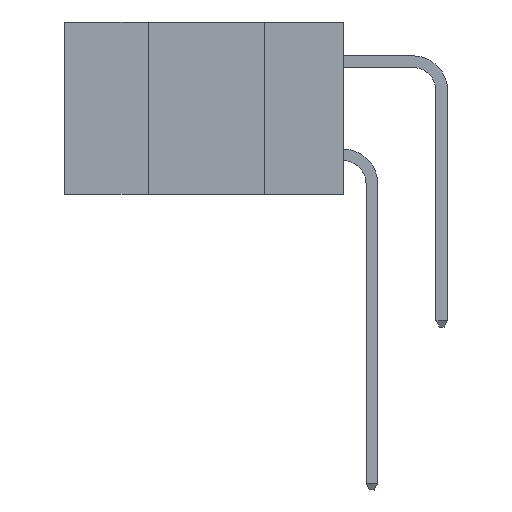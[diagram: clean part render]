
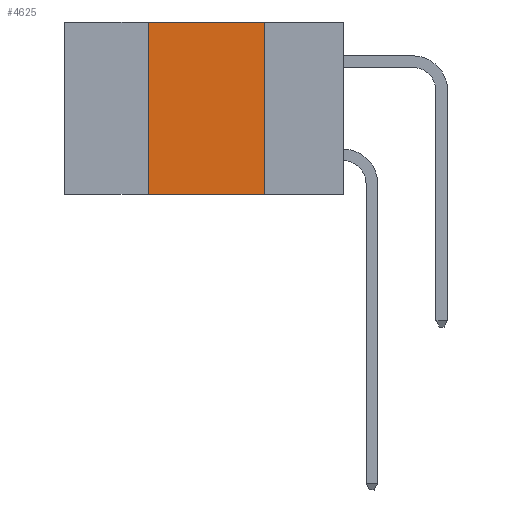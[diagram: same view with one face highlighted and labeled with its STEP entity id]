
A CAD part, left-side view. The second image highlights one B-rep face of the part: STEP entity #4625.
In plain terms, the highlighted planar face has unit normal (-1, 0, 0).
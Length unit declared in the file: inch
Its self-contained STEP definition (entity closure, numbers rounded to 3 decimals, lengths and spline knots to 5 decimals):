
#316 = LINE ( 'NONE', #6072, #7468 ) ;
#452 = EDGE_LOOP ( 'NONE', ( #10385, #9498, #10636, #984 ) ) ;
#498 = EDGE_CURVE ( 'NONE', #5081, #2629, #4426, .T. ) ;
#587 = CARTESIAN_POINT ( 'NONE',  ( 0., 0.42, 0. ) ) ;
#903 = DIRECTION ( 'NONE',  ( 1., 0., 0. ) ) ;
#962 = FACE_OUTER_BOUND ( 'NONE', #452, .T. ) ;
#984 = ORIENTED_EDGE ( 'NONE', *, *, #5746, .T. ) ;
#990 = CARTESIAN_POINT ( 'NONE',  ( 0., 0.6, 0. ) ) ;
#1086 = DIRECTION ( 'NONE',  ( 0., 0., -1. ) ) ;
#1478 = VECTOR ( 'NONE', #10584, 39.37008 ) ;
#1640 = PLANE ( 'NONE',  #8511 ) ;
#2348 = CARTESIAN_POINT ( 'NONE',  ( 0., 0.42, -0.37 ) ) ;
#2629 = VERTEX_POINT ( 'NONE', #8640 ) ;
#3432 = CARTESIAN_POINT ( 'NONE',  ( 0., 0.17, -0.37 ) ) ;
#3482 = CARTESIAN_POINT ( 'NONE',  ( 0., 0.6, -0.37 ) ) ;
#3766 = LINE ( 'NONE', #3482, #6515 ) ;
#3848 = CARTESIAN_POINT ( 'NONE',  ( 0., 0.42, 0. ) ) ;
#4426 = LINE ( 'NONE', #10821, #1478 ) ;
#4625 = ADVANCED_FACE ( 'NONE', ( #962 ), #1640, .F. ) ;
#5081 = VERTEX_POINT ( 'NONE', #587 ) ;
#5691 = VERTEX_POINT ( 'NONE', #2348 ) ;
#5729 = LINE ( 'NONE', #3848, #10146 ) ;
#5746 = EDGE_CURVE ( 'NONE', #5691, #7994, #3766, .T. ) ;
#6072 = CARTESIAN_POINT ( 'NONE',  ( 0., 0.17, 0. ) ) ;
#6515 = VECTOR ( 'NONE', #8318, 39.37008 ) ;
#7304 = DIRECTION ( 'NONE',  ( 0., 0., -1. ) ) ;
#7468 = VECTOR ( 'NONE', #1086, 39.37008 ) ;
#7586 = EDGE_CURVE ( 'NONE', #2629, #7994, #316, .T. ) ;
#7994 = VERTEX_POINT ( 'NONE', #3432 ) ;
#8316 = EDGE_CURVE ( 'NONE', #5691, #5081, #5729, .T. ) ;
#8318 = DIRECTION ( 'NONE',  ( 0., -1., 0. ) ) ;
#8511 = AXIS2_PLACEMENT_3D ( 'NONE', #990, #903, #7304 ) ;
#8640 = CARTESIAN_POINT ( 'NONE',  ( 0., 0.17, 0. ) ) ;
#9498 = ORIENTED_EDGE ( 'NONE', *, *, #498, .F. ) ;
#10146 = VECTOR ( 'NONE', #11159, 39.37008 ) ;
#10385 = ORIENTED_EDGE ( 'NONE', *, *, #7586, .F. ) ;
#10584 = DIRECTION ( 'NONE',  ( 0., -1., 0. ) ) ;
#10636 = ORIENTED_EDGE ( 'NONE', *, *, #8316, .F. ) ;
#10821 = CARTESIAN_POINT ( 'NONE',  ( 0., 0.6, 0. ) ) ;
#11159 = DIRECTION ( 'NONE',  ( 0., 0., 1. ) ) ;
